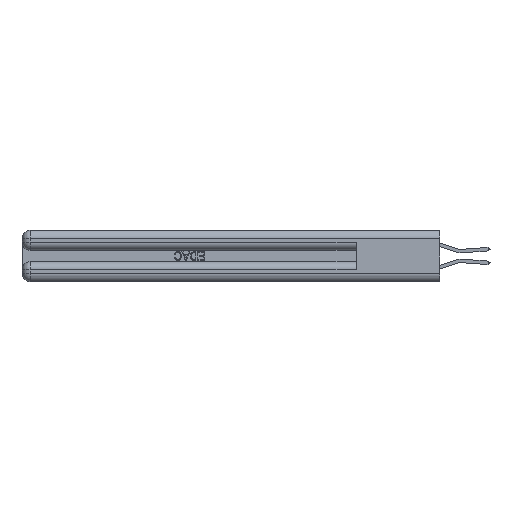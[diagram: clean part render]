
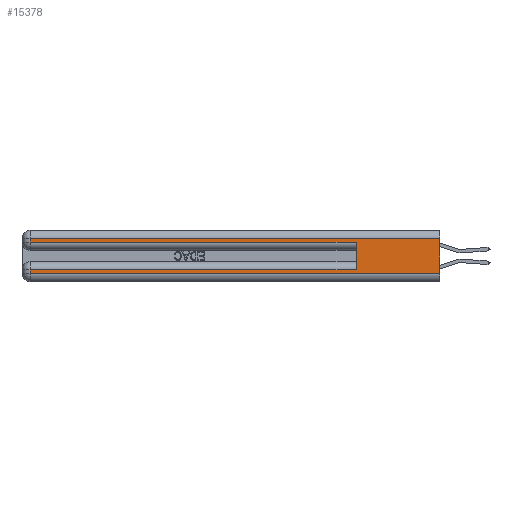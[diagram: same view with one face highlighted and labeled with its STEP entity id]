
A CAD part, left-side view. The second image highlights one B-rep face of the part: STEP entity #15378.
In plain terms, the highlighted planar face has unit normal (-1, 0, 0).
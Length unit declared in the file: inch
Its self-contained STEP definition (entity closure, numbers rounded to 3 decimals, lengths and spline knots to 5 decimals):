
#1467 = ORIENTED_EDGE ( 'NONE', *, *, #7191, .T. ) ;
#1809 = VERTEX_POINT ( 'NONE', #39707 ) ;
#2014 = VECTOR ( 'NONE', #20954, 39.37008 ) ;
#2799 = CARTESIAN_POINT ( 'NONE',  ( 0., 0., 0.06 ) ) ;
#3142 = EDGE_CURVE ( 'NONE', #39494, #1809, #12886, .T. ) ;
#5200 = DIRECTION ( 'NONE',  ( 0., 1., 0. ) ) ;
#5584 = ORIENTED_EDGE ( 'NONE', *, *, #13584, .T. ) ;
#5691 = EDGE_LOOP ( 'NONE', ( #23844, #42282, #20999, #6177, #41664, #5584, #6996, #1467 ) ) ;
#5700 = CARTESIAN_POINT ( 'NONE',  ( 0., 0.6, 0.145 ) ) ;
#5780 = LINE ( 'NONE', #37027, #15488 ) ;
#6177 = ORIENTED_EDGE ( 'NONE', *, *, #3142, .T. ) ;
#6342 = CARTESIAN_POINT ( 'NONE',  ( 0., 2.94, 0.37 ) ) ;
#6852 = VECTOR ( 'NONE', #20158, 39.37008 ) ;
#6996 = ORIENTED_EDGE ( 'NONE', *, *, #41899, .T. ) ;
#7191 = EDGE_CURVE ( 'NONE', #21960, #22165, #36741, .T. ) ;
#7692 = VERTEX_POINT ( 'NONE', #45149 ) ;
#7945 = VECTOR ( 'NONE', #21074, 39.37008 ) ;
#8169 = DIRECTION ( 'NONE',  ( 0., 1., 0. ) ) ;
#9044 = VERTEX_POINT ( 'NONE', #30224 ) ;
#11422 = VERTEX_POINT ( 'NONE', #17562 ) ;
#11729 = LINE ( 'NONE', #6342, #2014 ) ;
#11730 = VECTOR ( 'NONE', #21348, 39.37008 ) ;
#12038 = DIRECTION ( 'NONE',  ( 0., 0., -1. ) ) ;
#12886 = LINE ( 'NONE', #39196, #11730 ) ;
#13457 = DIRECTION ( 'NONE',  ( 0., 0., -1. ) ) ;
#13584 = EDGE_CURVE ( 'NONE', #35365, #7692, #41484, .T. ) ;
#15378 = ADVANCED_FACE ( 'NONE', ( #28636 ), #27783, .F. ) ;
#15488 = VECTOR ( 'NONE', #8169, 39.37008 ) ;
#16562 = LINE ( 'NONE', #5700, #6852 ) ;
#16957 = EDGE_CURVE ( 'NONE', #11422, #9044, #5780, .T. ) ;
#17562 = CARTESIAN_POINT ( 'NONE',  ( 0., 0., 0.31 ) ) ;
#19937 = CARTESIAN_POINT ( 'NONE',  ( 0., 0., 0.06 ) ) ;
#20158 = DIRECTION ( 'NONE',  ( 0., 0., 1. ) ) ;
#20954 = DIRECTION ( 'NONE',  ( 0., 0., -1. ) ) ;
#20999 = ORIENTED_EDGE ( 'NONE', *, *, #34651, .T. ) ;
#21074 = DIRECTION ( 'NONE',  ( 0., -1., 0. ) ) ;
#21319 = VECTOR ( 'NONE', #5200, 39.37008 ) ;
#21348 = DIRECTION ( 'NONE',  ( 0., -1., 0. ) ) ;
#21960 = VERTEX_POINT ( 'NONE', #40338 ) ;
#22165 = VERTEX_POINT ( 'NONE', #19937 ) ;
#23844 = ORIENTED_EDGE ( 'NONE', *, *, #29909, .F. ) ;
#24159 = CARTESIAN_POINT ( 'NONE',  ( 0., 2.94, 0.37 ) ) ;
#26919 = VECTOR ( 'NONE', #12038, 39.37008 ) ;
#27783 = PLANE ( 'NONE',  #34848 ) ;
#28636 = FACE_OUTER_BOUND ( 'NONE', #5691, .T. ) ;
#29909 = EDGE_CURVE ( 'NONE', #11422, #22165, #36440, .T. ) ;
#30224 = CARTESIAN_POINT ( 'NONE',  ( 0., 2.94, 0.31 ) ) ;
#31382 = CARTESIAN_POINT ( 'NONE',  ( 0., 0., 0.37 ) ) ;
#33377 = VECTOR ( 'NONE', #45593, 39.37008 ) ;
#34651 = EDGE_CURVE ( 'NONE', #9044, #39494, #41732, .T. ) ;
#34848 = AXIS2_PLACEMENT_3D ( 'NONE', #31382, #34989, #13457 ) ;
#34989 = DIRECTION ( 'NONE',  ( 1., 0., 0. ) ) ;
#35365 = VERTEX_POINT ( 'NONE', #45980 ) ;
#35585 = CARTESIAN_POINT ( 'NONE',  ( 0., 2.94, 0.285 ) ) ;
#36440 = LINE ( 'NONE', #40779, #26919 ) ;
#36741 = LINE ( 'NONE', #2799, #7945 ) ;
#37027 = CARTESIAN_POINT ( 'NONE',  ( 0., 0., 0.31 ) ) ;
#39196 = CARTESIAN_POINT ( 'NONE',  ( 0., 0., 0.285 ) ) ;
#39494 = VERTEX_POINT ( 'NONE', #35585 ) ;
#39707 = CARTESIAN_POINT ( 'NONE',  ( 0., 0.6, 0.285 ) ) ;
#40338 = CARTESIAN_POINT ( 'NONE',  ( 0., 2.94, 0.06 ) ) ;
#40779 = CARTESIAN_POINT ( 'NONE',  ( 0., 0., 0.37 ) ) ;
#41132 = CARTESIAN_POINT ( 'NONE',  ( 0., 0., 0.085 ) ) ;
#41484 = LINE ( 'NONE', #41132, #21319 ) ;
#41664 = ORIENTED_EDGE ( 'NONE', *, *, #45468, .F. ) ;
#41732 = LINE ( 'NONE', #24159, #33377 ) ;
#41899 = EDGE_CURVE ( 'NONE', #7692, #21960, #11729, .T. ) ;
#42282 = ORIENTED_EDGE ( 'NONE', *, *, #16957, .T. ) ;
#45149 = CARTESIAN_POINT ( 'NONE',  ( 0., 2.94, 0.085 ) ) ;
#45468 = EDGE_CURVE ( 'NONE', #35365, #1809, #16562, .T. ) ;
#45593 = DIRECTION ( 'NONE',  ( 0., 0., -1. ) ) ;
#45980 = CARTESIAN_POINT ( 'NONE',  ( 0., 0.6, 0.085 ) ) ;
